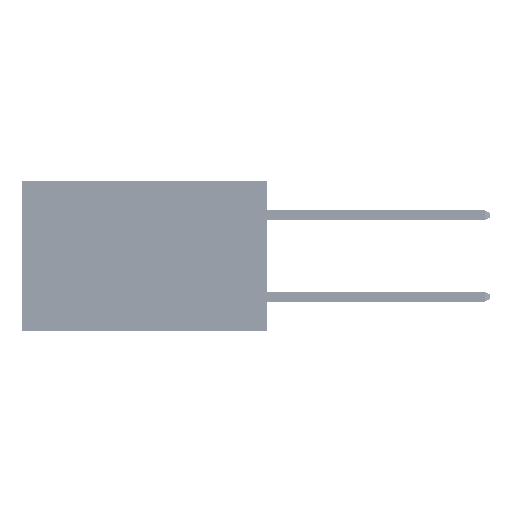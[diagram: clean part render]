
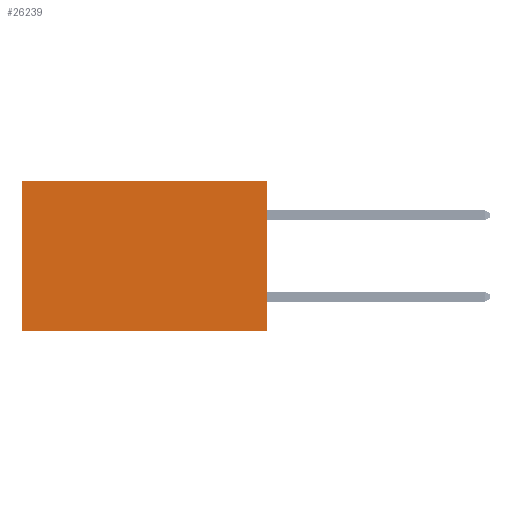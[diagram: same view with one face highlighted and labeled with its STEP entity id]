
A CAD part, left-side view. The second image highlights one B-rep face of the part: STEP entity #26239.
In plain terms, the highlighted planar face has unit normal (-1, 0, 0).
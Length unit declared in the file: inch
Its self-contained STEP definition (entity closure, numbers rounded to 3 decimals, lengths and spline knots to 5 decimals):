
#793 = CARTESIAN_POINT ( 'NONE',  ( 0.2875, 0.6, -0.37 ) ) ;
#1659 = ORIENTED_EDGE ( 'NONE', *, *, #22302, .F. ) ;
#2052 = PLANE ( 'NONE',  #46048 ) ;
#3814 = VERTEX_POINT ( 'NONE', #9513 ) ;
#4944 = CARTESIAN_POINT ( 'NONE',  ( 0.2875, 0., -0.37 ) ) ;
#7242 = VERTEX_POINT ( 'NONE', #4944 ) ;
#9201 = VECTOR ( 'NONE', #16831, 39.37008 ) ;
#9513 = CARTESIAN_POINT ( 'NONE',  ( 0.2875, 0.6, 0. ) ) ;
#9848 = ORIENTED_EDGE ( 'NONE', *, *, #34116, .F. ) ;
#10295 = CARTESIAN_POINT ( 'NONE',  ( 0.2875, 0., 0. ) ) ;
#10630 = DIRECTION ( 'NONE',  ( 0., 0., -1. ) ) ;
#11652 = VECTOR ( 'NONE', #30936, 39.37008 ) ;
#12670 = VECTOR ( 'NONE', #40232, 39.37008 ) ;
#14369 = LINE ( 'NONE', #18294, #12670 ) ;
#15741 = LINE ( 'NONE', #20184, #17985 ) ;
#16831 = DIRECTION ( 'NONE',  ( 0., 1., 0. ) ) ;
#17655 = CARTESIAN_POINT ( 'NONE',  ( 0.2875, 0., 0. ) ) ;
#17985 = VECTOR ( 'NONE', #45474, 39.37008 ) ;
#18294 = CARTESIAN_POINT ( 'NONE',  ( 0.2875, 0., -0.37 ) ) ;
#18834 = LINE ( 'NONE', #19700, #9201 ) ;
#19249 = EDGE_LOOP ( 'NONE', ( #43003, #1659, #9848, #41968 ) ) ;
#19700 = CARTESIAN_POINT ( 'NONE',  ( 0.2875, 0., 0. ) ) ;
#19744 = EDGE_CURVE ( 'NONE', #43739, #3814, #18834, .T. ) ;
#20184 = CARTESIAN_POINT ( 'NONE',  ( 0.2875, 0.6, 0. ) ) ;
#21193 = VERTEX_POINT ( 'NONE', #793 ) ;
#22302 = EDGE_CURVE ( 'NONE', #7242, #21193, #14369, .T. ) ;
#24144 = LINE ( 'NONE', #46009, #11652 ) ;
#25273 = DIRECTION ( 'NONE',  ( 1., 0., 0. ) ) ;
#25895 = FACE_OUTER_BOUND ( 'NONE', #19249, .T. ) ;
#26239 = ADVANCED_FACE ( 'NONE', ( #25895 ), #2052, .F. ) ;
#30936 = DIRECTION ( 'NONE',  ( 0., 0., -1. ) ) ;
#34116 = EDGE_CURVE ( 'NONE', #43739, #7242, #24144, .T. ) ;
#40232 = DIRECTION ( 'NONE',  ( 0., 1., 0. ) ) ;
#41027 = EDGE_CURVE ( 'NONE', #3814, #21193, #15741, .T. ) ;
#41968 = ORIENTED_EDGE ( 'NONE', *, *, #19744, .T. ) ;
#43003 = ORIENTED_EDGE ( 'NONE', *, *, #41027, .T. ) ;
#43739 = VERTEX_POINT ( 'NONE', #10295 ) ;
#45474 = DIRECTION ( 'NONE',  ( 0., 0., -1. ) ) ;
#46009 = CARTESIAN_POINT ( 'NONE',  ( 0.2875, 0., 0. ) ) ;
#46048 = AXIS2_PLACEMENT_3D ( 'NONE', #17655, #25273, #10630 ) ;
